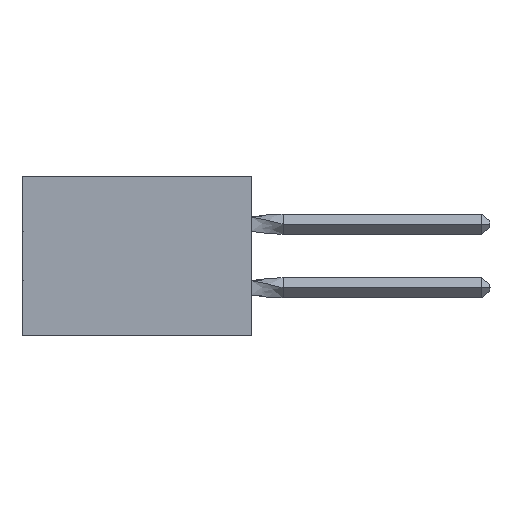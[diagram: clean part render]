
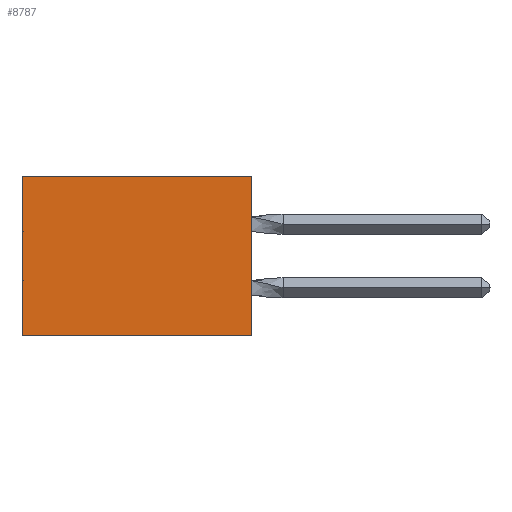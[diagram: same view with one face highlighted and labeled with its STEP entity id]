
A CAD part, left-side view. The second image highlights one B-rep face of the part: STEP entity #8787.
In plain terms, the highlighted planar face has unit normal (-1, 0, 0).
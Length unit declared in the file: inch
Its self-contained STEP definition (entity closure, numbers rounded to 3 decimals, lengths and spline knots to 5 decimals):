
#1598 = VECTOR ( 'NONE', #11546, 39.37008 ) ;
#1680 = EDGE_CURVE ( 'NONE', #9279, #44274, #46704, .T. ) ;
#2024 = CARTESIAN_POINT ( 'NONE',  ( 0.305, 0., -0.5 ) ) ;
#5161 = EDGE_CURVE ( 'NONE', #9279, #49034, #6681, .T. ) ;
#5877 = DIRECTION ( 'NONE',  ( 0., 0., -1. ) ) ;
#6681 = LINE ( 'NONE', #45896, #36143 ) ;
#8787 = ADVANCED_FACE ( 'NONE', ( #45707 ), #18211, .F. ) ;
#9279 = VERTEX_POINT ( 'NONE', #9538 ) ;
#9538 = CARTESIAN_POINT ( 'NONE',  ( 0.305, 0., 0. ) ) ;
#10072 = DIRECTION ( 'NONE',  ( 0., 0., -1. ) ) ;
#10167 = VERTEX_POINT ( 'NONE', #26074 ) ;
#11546 = DIRECTION ( 'NONE',  ( 0., 0., -1. ) ) ;
#11625 = DIRECTION ( 'NONE',  ( 0., 1., 0. ) ) ;
#15232 = EDGE_CURVE ( 'NONE', #44274, #10167, #37844, .T. ) ;
#16877 = VECTOR ( 'NONE', #11625, 39.37008 ) ;
#17827 = ORIENTED_EDGE ( 'NONE', *, *, #15232, .F. ) ;
#18211 = PLANE ( 'NONE',  #25200 ) ;
#22144 = CARTESIAN_POINT ( 'NONE',  ( 0.305, 0., -0.5 ) ) ;
#22565 = CARTESIAN_POINT ( 'NONE',  ( 0.305, 0., -0.5 ) ) ;
#23440 = DIRECTION ( 'NONE',  ( 0., 1., 0. ) ) ;
#25200 = AXIS2_PLACEMENT_3D ( 'NONE', #2024, #28929, #5877 ) ;
#26074 = CARTESIAN_POINT ( 'NONE',  ( 0.305, 0.72, -0.5 ) ) ;
#28929 = DIRECTION ( 'NONE',  ( 1., 0., 0. ) ) ;
#31741 = CARTESIAN_POINT ( 'NONE',  ( 0.305, 0., -0.5 ) ) ;
#33379 = EDGE_CURVE ( 'NONE', #49034, #10167, #44430, .T. ) ;
#33580 = VECTOR ( 'NONE', #10072, 39.37008 ) ;
#33826 = ORIENTED_EDGE ( 'NONE', *, *, #5161, .T. ) ;
#36143 = VECTOR ( 'NONE', #23440, 39.37008 ) ;
#36963 = ORIENTED_EDGE ( 'NONE', *, *, #1680, .F. ) ;
#37844 = LINE ( 'NONE', #22144, #16877 ) ;
#40289 = CARTESIAN_POINT ( 'NONE',  ( 0.305, 0.72, 0. ) ) ;
#44274 = VERTEX_POINT ( 'NONE', #31741 ) ;
#44430 = LINE ( 'NONE', #48221, #33580 ) ;
#45707 = FACE_OUTER_BOUND ( 'NONE', #48083, .T. ) ;
#45896 = CARTESIAN_POINT ( 'NONE',  ( 0.305, 0., 0. ) ) ;
#46704 = LINE ( 'NONE', #22565, #1598 ) ;
#48083 = EDGE_LOOP ( 'NONE', ( #49254, #17827, #36963, #33826 ) ) ;
#48221 = CARTESIAN_POINT ( 'NONE',  ( 0.305, 0.72, -0.5 ) ) ;
#49034 = VERTEX_POINT ( 'NONE', #40289 ) ;
#49254 = ORIENTED_EDGE ( 'NONE', *, *, #33379, .T. ) ;
